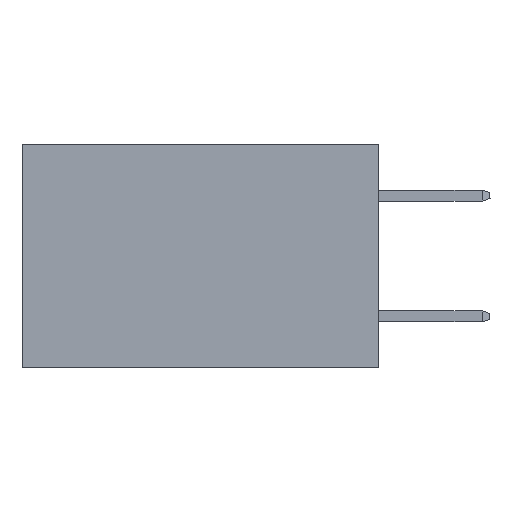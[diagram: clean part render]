
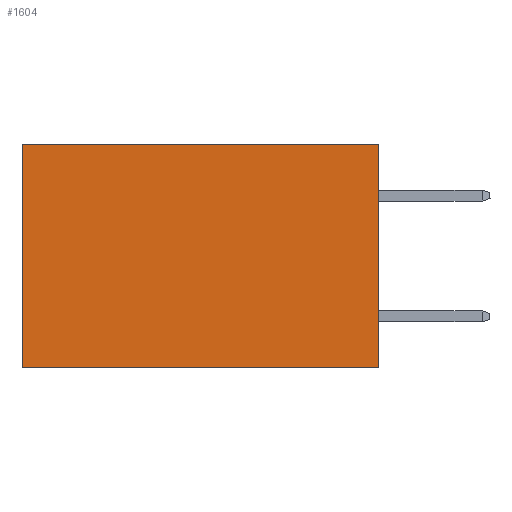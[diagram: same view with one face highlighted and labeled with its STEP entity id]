
A CAD part, left-side view. The second image highlights one B-rep face of the part: STEP entity #1604.
In plain terms, the highlighted planar face has unit normal (-1, 0, 0).
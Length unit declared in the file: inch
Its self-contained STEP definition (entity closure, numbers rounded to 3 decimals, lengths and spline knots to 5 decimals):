
#287 = CARTESIAN_POINT ( 'NONE',  ( 0.277, 0., -0.37 ) ) ;
#1056 = DIRECTION ( 'NONE',  ( 0., 0., -1. ) ) ;
#1134 = ORIENTED_EDGE ( 'NONE', *, *, #3495, .F. ) ;
#1165 = DIRECTION ( 'NONE',  ( 0., 0., -1. ) ) ;
#1604 = ADVANCED_FACE ( 'NONE', ( #12258 ), #1905, .F. ) ;
#1867 = VERTEX_POINT ( 'NONE', #4669 ) ;
#1905 = PLANE ( 'NONE',  #3273 ) ;
#1913 = CARTESIAN_POINT ( 'NONE',  ( 0.277, 0., -0.37 ) ) ;
#1982 = DIRECTION ( 'NONE',  ( 1., 0., 0. ) ) ;
#2748 = CARTESIAN_POINT ( 'NONE',  ( 0.277, 0.59, 0. ) ) ;
#3042 = VECTOR ( 'NONE', #10915, 39.37008 ) ;
#3273 = AXIS2_PLACEMENT_3D ( 'NONE', #1913, #1982, #1165 ) ;
#3495 = EDGE_CURVE ( 'NONE', #13235, #1867, #7626, .T. ) ;
#3673 = ORIENTED_EDGE ( 'NONE', *, *, #10791, .F. ) ;
#4381 = VECTOR ( 'NONE', #1056, 39.37008 ) ;
#4669 = CARTESIAN_POINT ( 'NONE',  ( 0.277, 0., -0.37 ) ) ;
#5005 = LINE ( 'NONE', #7215, #5391 ) ;
#5391 = VECTOR ( 'NONE', #14490, 39.37008 ) ;
#7215 = CARTESIAN_POINT ( 'NONE',  ( 0.277, 0.59, -0.37 ) ) ;
#7452 = EDGE_CURVE ( 'NONE', #9937, #8359, #5005, .T. ) ;
#7626 = LINE ( 'NONE', #287, #4381 ) ;
#8359 = VERTEX_POINT ( 'NONE', #13625 ) ;
#8901 = LINE ( 'NONE', #11665, #14978 ) ;
#9937 = VERTEX_POINT ( 'NONE', #2748 ) ;
#10403 = CARTESIAN_POINT ( 'NONE',  ( 0.277, 0., 0. ) ) ;
#10791 = EDGE_CURVE ( 'NONE', #1867, #8359, #8901, .T. ) ;
#10915 = DIRECTION ( 'NONE',  ( 0., 1., 0. ) ) ;
#11665 = CARTESIAN_POINT ( 'NONE',  ( 0.277, 0., -0.37 ) ) ;
#11784 = EDGE_LOOP ( 'NONE', ( #12659, #3673, #1134, #14177 ) ) ;
#12258 = FACE_OUTER_BOUND ( 'NONE', #11784, .T. ) ;
#12659 = ORIENTED_EDGE ( 'NONE', *, *, #7452, .T. ) ;
#12881 = DIRECTION ( 'NONE',  ( 0., 1., 0. ) ) ;
#13235 = VERTEX_POINT ( 'NONE', #10403 ) ;
#13352 = CARTESIAN_POINT ( 'NONE',  ( 0.277, 0., 0. ) ) ;
#13625 = CARTESIAN_POINT ( 'NONE',  ( 0.277, 0.59, -0.37 ) ) ;
#14177 = ORIENTED_EDGE ( 'NONE', *, *, #15512, .T. ) ;
#14490 = DIRECTION ( 'NONE',  ( 0., 0., -1. ) ) ;
#14978 = VECTOR ( 'NONE', #12881, 39.37008 ) ;
#15512 = EDGE_CURVE ( 'NONE', #13235, #9937, #15648, .T. ) ;
#15648 = LINE ( 'NONE', #13352, #3042 ) ;
